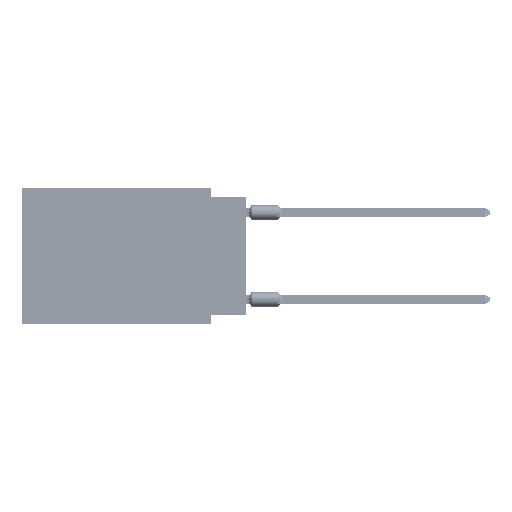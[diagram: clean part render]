
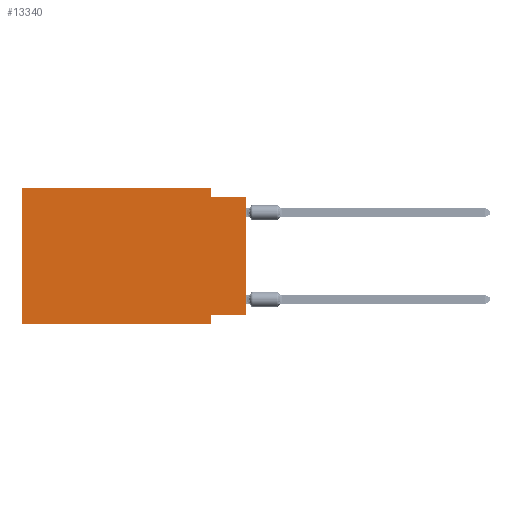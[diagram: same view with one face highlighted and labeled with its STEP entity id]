
A CAD part, left-side view. The second image highlights one B-rep face of the part: STEP entity #13340.
In plain terms, the highlighted planar face has unit normal (-1, 0, 0).
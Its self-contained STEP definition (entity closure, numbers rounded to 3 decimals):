
#3579 = AXIS2_PLACEMENT_3D ( 'NONE', #10985, #39643, #76850 ) ;
#3911 = ORIENTED_EDGE ( 'NONE', *, *, #70983, .F. ) ;
#5234 = VERTEX_POINT ( 'NONE', #10382 ) ;
#6076 = LINE ( 'NONE', #41418, #68706 ) ;
#8441 = CARTESIAN_POINT ( 'NONE',  ( 0., 16.383, -9.906 ) ) ;
#9217 = DIRECTION ( 'NONE',  ( 0., 0., -1. ) ) ;
#10382 = CARTESIAN_POINT ( 'NONE',  ( 0., 2.54, -0.635 ) ) ;
#10985 = CARTESIAN_POINT ( 'NONE',  ( 0., 16.383, 0. ) ) ;
#11749 = VERTEX_POINT ( 'NONE', #15209 ) ;
#11791 = EDGE_CURVE ( 'NONE', #5234, #74279, #62671, .T. ) ;
#13283 = EDGE_CURVE ( 'NONE', #75983, #55129, #14129, .T. ) ;
#13340 = ADVANCED_FACE ( 'NONE', ( #45516 ), #70576, .F. ) ;
#13872 = EDGE_LOOP ( 'NONE', ( #54128, #28831, #29522, #25680, #39251, #22244, #3911, #57853 ) ) ;
#14129 = LINE ( 'NONE', #20812, #22304 ) ;
#15091 = LINE ( 'NONE', #39038, #65402 ) ;
#15209 = CARTESIAN_POINT ( 'NONE',  ( 0., 0., -9.271 ) ) ;
#15997 = CARTESIAN_POINT ( 'NONE',  ( 0., 0., -9.271 ) ) ;
#16657 = LINE ( 'NONE', #35127, #48746 ) ;
#17563 = CARTESIAN_POINT ( 'NONE',  ( 0., 16.383, 0. ) ) ;
#17744 = VERTEX_POINT ( 'NONE', #19127 ) ;
#19127 = CARTESIAN_POINT ( 'NONE',  ( 0., 16.383, 0. ) ) ;
#20333 = DIRECTION ( 'NONE',  ( 0., -1., 0. ) ) ;
#20678 = VECTOR ( 'NONE', #40345, 1000. ) ;
#20812 = CARTESIAN_POINT ( 'NONE',  ( 0., 16.383, -9.906 ) ) ;
#21230 = CARTESIAN_POINT ( 'NONE',  ( 0., 2.54, -9.906 ) ) ;
#22244 = ORIENTED_EDGE ( 'NONE', *, *, #13283, .T. ) ;
#22304 = VECTOR ( 'NONE', #73345, 1000. ) ;
#22724 = VERTEX_POINT ( 'NONE', #60709 ) ;
#23448 = LINE ( 'NONE', #17563, #53623 ) ;
#25680 = ORIENTED_EDGE ( 'NONE', *, *, #74856, .F. ) ;
#27318 = EDGE_CURVE ( 'NONE', #11749, #74279, #16657, .T. ) ;
#27746 = VECTOR ( 'NONE', #63675, 1000. ) ;
#28831 = ORIENTED_EDGE ( 'NONE', *, *, #11791, .F. ) ;
#29522 = ORIENTED_EDGE ( 'NONE', *, *, #32623, .F. ) ;
#30300 = CARTESIAN_POINT ( 'NONE',  ( 0., 2.54, 0. ) ) ;
#30374 = DIRECTION ( 'NONE',  ( 0., 0., -1. ) ) ;
#32623 = EDGE_CURVE ( 'NONE', #65395, #5234, #15091, .T. ) ;
#32895 = CARTESIAN_POINT ( 'NONE',  ( 0., 0., -0.635 ) ) ;
#35127 = CARTESIAN_POINT ( 'NONE',  ( 0., 0., 0. ) ) ;
#36425 = CARTESIAN_POINT ( 'NONE',  ( 0., 0., -0.635 ) ) ;
#39038 = CARTESIAN_POINT ( 'NONE',  ( 0., 2.54, 0. ) ) ;
#39165 = VECTOR ( 'NONE', #20333, 1000. ) ;
#39251 = ORIENTED_EDGE ( 'NONE', *, *, #54456, .F. ) ;
#39643 = DIRECTION ( 'NONE',  ( 1., 0., 0. ) ) ;
#40345 = DIRECTION ( 'NONE',  ( 0., 1., 0. ) ) ;
#40620 = DIRECTION ( 'NONE',  ( 0., 0., 1. ) ) ;
#41418 = CARTESIAN_POINT ( 'NONE',  ( 0., 2.54, -9.906 ) ) ;
#45516 = FACE_OUTER_BOUND ( 'NONE', #13872, .T. ) ;
#48746 = VECTOR ( 'NONE', #40620, 1000. ) ;
#53623 = VECTOR ( 'NONE', #72694, 1000. ) ;
#54128 = ORIENTED_EDGE ( 'NONE', *, *, #27318, .T. ) ;
#54456 = EDGE_CURVE ( 'NONE', #75983, #17744, #23448, .T. ) ;
#55129 = VERTEX_POINT ( 'NONE', #21230 ) ;
#57853 = ORIENTED_EDGE ( 'NONE', *, *, #63187, .F. ) ;
#60709 = CARTESIAN_POINT ( 'NONE',  ( 0., 2.54, -9.271 ) ) ;
#62671 = LINE ( 'NONE', #32895, #39165 ) ;
#63187 = EDGE_CURVE ( 'NONE', #11749, #22724, #75198, .T. ) ;
#63675 = DIRECTION ( 'NONE',  ( 0., -1., 0. ) ) ;
#65395 = VERTEX_POINT ( 'NONE', #30300 ) ;
#65402 = VECTOR ( 'NONE', #9217, 1000. ) ;
#68706 = VECTOR ( 'NONE', #30374, 1000. ) ;
#69172 = CARTESIAN_POINT ( 'NONE',  ( 0., 16.383, 0. ) ) ;
#69559 = LINE ( 'NONE', #69172, #27746 ) ;
#70576 = PLANE ( 'NONE',  #3579 ) ;
#70983 = EDGE_CURVE ( 'NONE', #22724, #55129, #6076, .T. ) ;
#72694 = DIRECTION ( 'NONE',  ( 0., 0., 1. ) ) ;
#73345 = DIRECTION ( 'NONE',  ( 0., -1., 0. ) ) ;
#74279 = VERTEX_POINT ( 'NONE', #36425 ) ;
#74856 = EDGE_CURVE ( 'NONE', #17744, #65395, #69559, .T. ) ;
#75198 = LINE ( 'NONE', #15997, #20678 ) ;
#75983 = VERTEX_POINT ( 'NONE', #8441 ) ;
#76850 = DIRECTION ( 'NONE',  ( 0., 0., -1. ) ) ;
